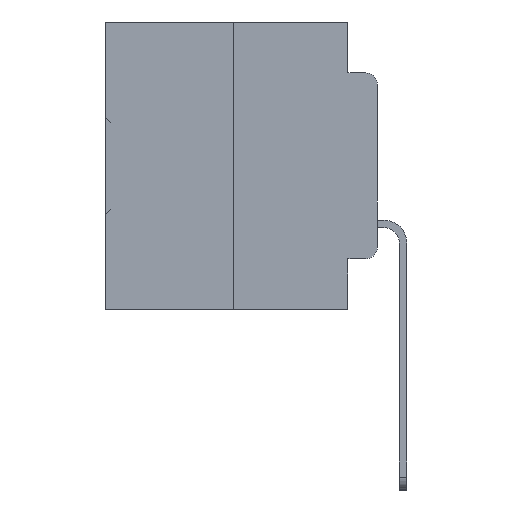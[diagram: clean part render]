
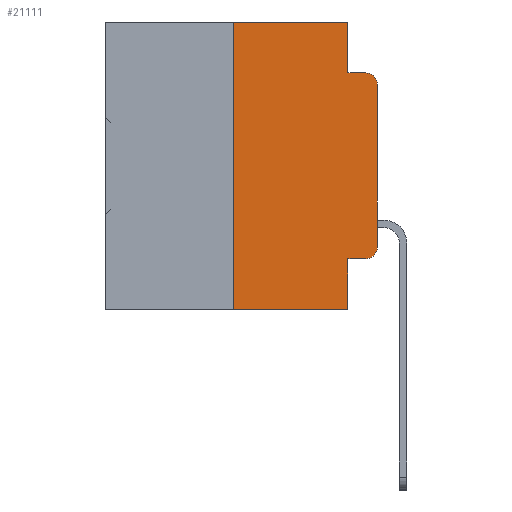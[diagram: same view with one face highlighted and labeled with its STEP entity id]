
A CAD part, left-side view. The second image highlights one B-rep face of the part: STEP entity #21111.
In plain terms, the highlighted planar face has unit normal (-1, 0, 0).
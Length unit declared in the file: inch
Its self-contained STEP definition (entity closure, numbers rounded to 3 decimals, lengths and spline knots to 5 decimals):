
#423 = VERTEX_POINT ( 'NONE', #19682 ) ;
#715 = CARTESIAN_POINT ( 'NONE',  ( 0., 0.051, 0. ) ) ;
#985 = EDGE_CURVE ( 'NONE', #20172, #423, #33512, .T. ) ;
#999 = CARTESIAN_POINT ( 'NONE',  ( 0., 0.473, 0. ) ) ;
#1776 = VERTEX_POINT ( 'NONE', #22904 ) ;
#2294 = LINE ( 'NONE', #10966, #30971 ) ;
#2380 = ORIENTED_EDGE ( 'NONE', *, *, #28625, .T. ) ;
#2445 = VECTOR ( 'NONE', #12941, 39.37008 ) ;
#2831 = ORIENTED_EDGE ( 'NONE', *, *, #24356, .F. ) ;
#3180 = CARTESIAN_POINT ( 'NONE',  ( 0., 0.02, -0.3915 ) ) ;
#3220 = VECTOR ( 'NONE', #7457, 39.37008 ) ;
#4222 = CARTESIAN_POINT ( 'NONE',  ( 0., 0.051, -0.4115 ) ) ;
#4420 = DIRECTION ( 'NONE',  ( -1., 0., 0. ) ) ;
#4938 = EDGE_CURVE ( 'NONE', #423, #23287, #30734, .T. ) ;
#5662 = EDGE_CURVE ( 'NONE', #1776, #13570, #11902, .T. ) ;
#7457 = DIRECTION ( 'NONE',  ( 0., -1., 0. ) ) ;
#7556 = CARTESIAN_POINT ( 'NONE',  ( 0., 0.051, -0.5 ) ) ;
#7567 = CARTESIAN_POINT ( 'NONE',  ( 0., 0.25, 0. ) ) ;
#7804 = ORIENTED_EDGE ( 'NONE', *, *, #4938, .T. ) ;
#8744 = VERTEX_POINT ( 'NONE', #7556 ) ;
#10966 = CARTESIAN_POINT ( 'NONE',  ( 0., 0.473, -0.5 ) ) ;
#11209 = LINE ( 'NONE', #31425, #32990 ) ;
#11843 = ORIENTED_EDGE ( 'NONE', *, *, #14028, .T. ) ;
#11902 = LINE ( 'NONE', #23735, #2445 ) ;
#12341 = DIRECTION ( 'NONE',  ( 0., 0., 1. ) ) ;
#12626 = DIRECTION ( 'NONE',  ( 1., 0., 0. ) ) ;
#12812 = DIRECTION ( 'NONE',  ( 0., 0., 1. ) ) ;
#12941 = DIRECTION ( 'NONE',  ( 0., -1., 0. ) ) ;
#13211 = VERTEX_POINT ( 'NONE', #20692 ) ;
#13213 = DIRECTION ( 'NONE',  ( 0., 0., -1. ) ) ;
#13570 = VERTEX_POINT ( 'NONE', #29552 ) ;
#13656 = LINE ( 'NONE', #31855, #25640 ) ;
#14028 = EDGE_CURVE ( 'NONE', #23287, #32126, #13656, .T. ) ;
#15194 = EDGE_CURVE ( 'NONE', #18956, #1776, #19880, .T. ) ;
#17158 = AXIS2_PLACEMENT_3D ( 'NONE', #21276, #4420, #24010 ) ;
#17733 = AXIS2_PLACEMENT_3D ( 'NONE', #3180, #32075, #26572 ) ;
#18205 = CARTESIAN_POINT ( 'NONE',  ( 0., 0.051, 0. ) ) ;
#18602 = EDGE_CURVE ( 'NONE', #13211, #8744, #2294, .T. ) ;
#18956 = VERTEX_POINT ( 'NONE', #18205 ) ;
#19682 = CARTESIAN_POINT ( 'NONE',  ( 0., 0.02, -0.4115 ) ) ;
#19880 = LINE ( 'NONE', #21284, #34214 ) ;
#20003 = AXIS2_PLACEMENT_3D ( 'NONE', #999, #12626, #31676 ) ;
#20172 = VERTEX_POINT ( 'NONE', #26730 ) ;
#20560 = CIRCLE ( 'NONE', #17158, 0.02 ) ;
#20692 = CARTESIAN_POINT ( 'NONE',  ( 0., 0.25, -0.5 ) ) ;
#21111 = ADVANCED_FACE ( 'NONE', ( #33531 ), #31562, .F. ) ;
#21276 = CARTESIAN_POINT ( 'NONE',  ( 0., 0.02, -0.1085 ) ) ;
#21284 = CARTESIAN_POINT ( 'NONE',  ( 0., 0.051, 0. ) ) ;
#21329 = ORIENTED_EDGE ( 'NONE', *, *, #23152, .F. ) ;
#22594 = EDGE_CURVE ( 'NONE', #13211, #31442, #11209, .T. ) ;
#22904 = CARTESIAN_POINT ( 'NONE',  ( 0., 0.051, -0.0885 ) ) ;
#23074 = ORIENTED_EDGE ( 'NONE', *, *, #5662, .F. ) ;
#23152 = EDGE_CURVE ( 'NONE', #31442, #18956, #27890, .T. ) ;
#23287 = VERTEX_POINT ( 'NONE', #35007 ) ;
#23489 = ORIENTED_EDGE ( 'NONE', *, *, #985, .T. ) ;
#23735 = CARTESIAN_POINT ( 'NONE',  ( 0., 0.051, -0.0885 ) ) ;
#23929 = EDGE_LOOP ( 'NONE', ( #11843, #2380, #23074, #35655, #21329, #25982, #29769, #2831, #23489, #7804 ) ) ;
#24010 = DIRECTION ( 'NONE',  ( 0., 0., -1. ) ) ;
#24356 = EDGE_CURVE ( 'NONE', #20172, #8744, #31145, .T. ) ;
#25640 = VECTOR ( 'NONE', #12812, 39.37008 ) ;
#25982 = ORIENTED_EDGE ( 'NONE', *, *, #22594, .F. ) ;
#26438 = CARTESIAN_POINT ( 'NONE',  ( 0., 0.473, 0. ) ) ;
#26572 = DIRECTION ( 'NONE',  ( 0., 0., -1. ) ) ;
#26730 = CARTESIAN_POINT ( 'NONE',  ( 0., 0.051, -0.4115 ) ) ;
#27491 = CARTESIAN_POINT ( 'NONE',  ( 0., 0., -0.1085 ) ) ;
#27890 = LINE ( 'NONE', #26438, #35015 ) ;
#28625 = EDGE_CURVE ( 'NONE', #32126, #13570, #20560, .T. ) ;
#29449 = VECTOR ( 'NONE', #31311, 39.37008 ) ;
#29552 = CARTESIAN_POINT ( 'NONE',  ( 0., 0.02, -0.0885 ) ) ;
#29769 = ORIENTED_EDGE ( 'NONE', *, *, #18602, .T. ) ;
#30107 = DIRECTION ( 'NONE',  ( 0., -1., 0. ) ) ;
#30734 = CIRCLE ( 'NONE', #17733, 0.02 ) ;
#30971 = VECTOR ( 'NONE', #30107, 39.37008 ) ;
#31145 = LINE ( 'NONE', #715, #29449 ) ;
#31311 = DIRECTION ( 'NONE',  ( 0., 0., -1. ) ) ;
#31425 = CARTESIAN_POINT ( 'NONE',  ( 0., 0.25, 0. ) ) ;
#31442 = VERTEX_POINT ( 'NONE', #7567 ) ;
#31562 = PLANE ( 'NONE',  #20003 ) ;
#31676 = DIRECTION ( 'NONE',  ( 0., 0., -1. ) ) ;
#31725 = DIRECTION ( 'NONE',  ( 0., -1., 0. ) ) ;
#31855 = CARTESIAN_POINT ( 'NONE',  ( 0., 0., 0. ) ) ;
#32075 = DIRECTION ( 'NONE',  ( -1., 0., 0. ) ) ;
#32126 = VERTEX_POINT ( 'NONE', #27491 ) ;
#32990 = VECTOR ( 'NONE', #12341, 39.37008 ) ;
#33512 = LINE ( 'NONE', #4222, #3220 ) ;
#33531 = FACE_OUTER_BOUND ( 'NONE', #23929, .T. ) ;
#34214 = VECTOR ( 'NONE', #13213, 39.37008 ) ;
#35007 = CARTESIAN_POINT ( 'NONE',  ( 0., 0., -0.3915 ) ) ;
#35015 = VECTOR ( 'NONE', #31725, 39.37008 ) ;
#35655 = ORIENTED_EDGE ( 'NONE', *, *, #15194, .F. ) ;
